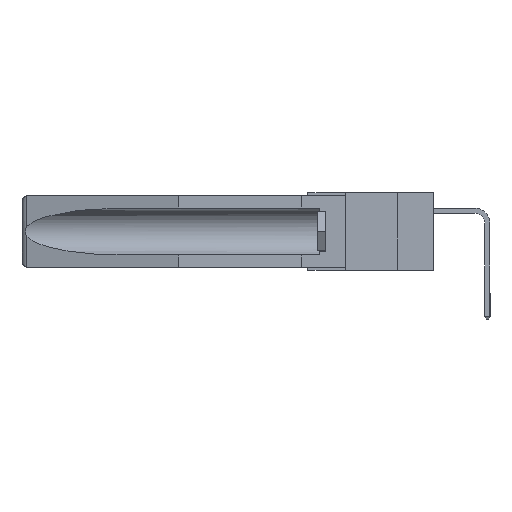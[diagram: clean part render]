
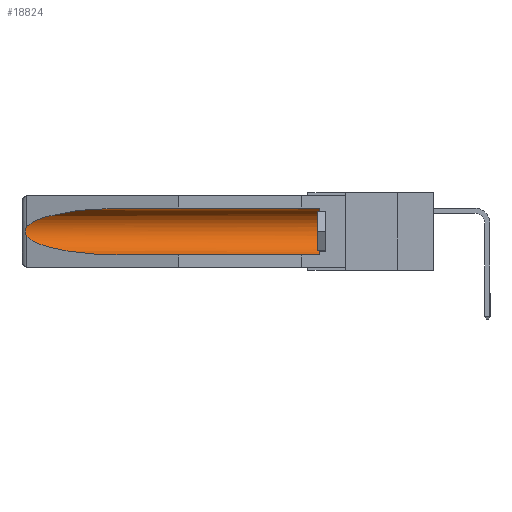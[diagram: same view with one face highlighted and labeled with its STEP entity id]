
A CAD part, left-side view. The second image highlights one B-rep face of the part: STEP entity #18824.
In plain terms, the highlighted cylindrical face has radius 2.857 mm (diameter 5.715 mm), a partial arc.
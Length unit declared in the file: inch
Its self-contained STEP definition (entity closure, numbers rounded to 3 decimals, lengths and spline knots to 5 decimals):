
#1118 = DIRECTION ( 'NONE',  ( 0., 1., 0. ) ) ;
#1363 = CARTESIAN_POINT ( 'NONE',  ( 0.26537, 1.52718, -0.19328 ) ) ;
#1457 = CARTESIAN_POINT ( 'NONE',  ( 0.25451, 1.48313, -0.24835 ) ) ;
#1878 = EDGE_CURVE ( 'NONE', #3964, #5398, #10526, .T. ) ;
#2089 = CARTESIAN_POINT ( 'NONE',  ( 0.26537, 1.52718, -0.19328 ) ) ;
#2339 = CARTESIAN_POINT ( 'NONE',  ( 0.26597, 1.5296, -0.19026 ) ) ;
#2630 = LINE ( 'NONE', #3405, #18219 ) ;
#3106 = VERTEX_POINT ( 'NONE', #24702 ) ;
#3405 = CARTESIAN_POINT ( 'NONE',  ( 0.155, -0.30754, -0.284 ) ) ;
#3619 = B_SPLINE_CURVE_WITH_KNOTS ( 'NONE', 3,
 ( #24090, #20144, #16199, #22167, #8186, #16105, #10196, #6261, #2339, #22258 ),
 .UNSPECIFIED., .F., .F.,
 ( 4, 2, 2, 2, 4 ),
 ( 0., 0.00029, 0.00058, 0.00087, 0.00117 ),
 .UNSPECIFIED. ) ;
#3673 = CARTESIAN_POINT ( 'NONE',  ( 0.155, 1.07973, -0.284 ) ) ;
#3964 = VERTEX_POINT ( 'NONE', #5039 ) ;
#5039 = CARTESIAN_POINT ( 'NONE',  ( 0.155, 1.07973, -0.059 ) ) ;
#5398 = VERTEX_POINT ( 'NONE', #8297 ) ;
#5708 = AXIS2_PLACEMENT_3D ( 'NONE', #14199, #18314, #12189 ) ;
#6104 = CYLINDRICAL_SURFACE ( 'NONE', #22093, 0.1125 ) ;
#6261 = CARTESIAN_POINT ( 'NONE',  ( 0.26655, 1.53094, -0.18657 ) ) ;
#6269 = CARTESIAN_POINT ( 'NONE',  ( 0.21114, 1.30732, -0.059 ) ) ;
#6389 = CARTESIAN_POINT ( 'NONE',  ( 0.155, -0.30754, -0.059 ) ) ;
#6666 =( BOUNDED_CURVE ( )  B_SPLINE_CURVE ( 3, ( #1363, #1457, #25586, #3673 ),
 .UNSPECIFIED., .F., .F. ) 
 B_SPLINE_CURVE_WITH_KNOTS ( ( 4, 4 ),
 ( 0.1948, 1.5708 ),
 .UNSPECIFIED. ) 
 CURVE ( )  GEOMETRIC_REPRESENTATION_ITEM ( )  RATIONAL_B_SPLINE_CURVE ( ( 1., 0.848, 0.848, 1. ) ) 
 REPRESENTATION_ITEM ( '' )  );
#7310 = DIRECTION ( 'NONE',  ( 0., 1., 0. ) ) ;
#8186 = CARTESIAN_POINT ( 'NONE',  ( 0.2675, 1.53308, -0.16763 ) ) ;
#8297 = CARTESIAN_POINT ( 'NONE',  ( 0.26537, 1.52718, -0.14972 ) ) ;
#8419 = DIRECTION ( 'NONE',  ( 0., 1., 0. ) ) ;
#8930 = FACE_OUTER_BOUND ( 'NONE', #15520, .T. ) ;
#9286 = ORIENTED_EDGE ( 'NONE', *, *, #22176, .T. ) ;
#10196 = CARTESIAN_POINT ( 'NONE',  ( 0.2673, 1.53269, -0.17917 ) ) ;
#10303 = CARTESIAN_POINT ( 'NONE',  ( 0.25451, 1.48313, -0.09465 ) ) ;
#10526 =( BOUNDED_CURVE ( )  B_SPLINE_CURVE ( 3, ( #21999, #6269, #10303, #11955 ),
 .UNSPECIFIED., .F., .F. ) 
 B_SPLINE_CURVE_WITH_KNOTS ( ( 4, 4 ),
 ( 4.71239, 6.08839 ),
 .UNSPECIFIED. ) 
 CURVE ( )  GEOMETRIC_REPRESENTATION_ITEM ( )  RATIONAL_B_SPLINE_CURVE ( ( 1., 0.848, 0.848, 1. ) ) 
 REPRESENTATION_ITEM ( '' )  );
#10573 = ORIENTED_EDGE ( 'NONE', *, *, #18373, .F. ) ;
#11500 = LINE ( 'NONE', #6389, #14938 ) ;
#11955 = CARTESIAN_POINT ( 'NONE',  ( 0.26537, 1.52718, -0.14972 ) ) ;
#12189 = DIRECTION ( 'NONE',  ( 0., 0., 1. ) ) ;
#12493 = EDGE_CURVE ( 'NONE', #25366, #17667, #6666, .T. ) ;
#12933 = EDGE_CURVE ( 'NONE', #3106, #3964, #11500, .T. ) ;
#14199 = CARTESIAN_POINT ( 'NONE',  ( 0.155, 0.126, -0.1715 ) ) ;
#14256 = ORIENTED_EDGE ( 'NONE', *, *, #12933, .T. ) ;
#14938 = VECTOR ( 'NONE', #8419, 39.37008 ) ;
#15520 = EDGE_LOOP ( 'NONE', ( #18788, #9286, #17429, #10573, #16141, #14256 ) ) ;
#16105 = CARTESIAN_POINT ( 'NONE',  ( 0.2675, 1.53308, -0.17534 ) ) ;
#16141 = ORIENTED_EDGE ( 'NONE', *, *, #20660, .T. ) ;
#16199 = CARTESIAN_POINT ( 'NONE',  ( 0.26654, 1.53092, -0.15636 ) ) ;
#17298 = CARTESIAN_POINT ( 'NONE',  ( 0.155, 0.126, -0.284 ) ) ;
#17429 = ORIENTED_EDGE ( 'NONE', *, *, #12493, .T. ) ;
#17509 = CIRCLE ( 'NONE', #5708, 0.1125 ) ;
#17667 = VERTEX_POINT ( 'NONE', #23056 ) ;
#17870 = VERTEX_POINT ( 'NONE', #17298 ) ;
#18219 = VECTOR ( 'NONE', #7310, 39.37008 ) ;
#18314 = DIRECTION ( 'NONE',  ( 0., -1., 0. ) ) ;
#18373 = EDGE_CURVE ( 'NONE', #17870, #17667, #2630, .T. ) ;
#18788 = ORIENTED_EDGE ( 'NONE', *, *, #1878, .T. ) ;
#18824 = ADVANCED_FACE ( 'NONE', ( #8930 ), #6104, .F. ) ;
#20144 = CARTESIAN_POINT ( 'NONE',  ( 0.26597, 1.52961, -0.15275 ) ) ;
#20660 = EDGE_CURVE ( 'NONE', #17870, #3106, #17509, .T. ) ;
#21772 = DIRECTION ( 'NONE',  ( 0., 0., 1. ) ) ;
#21999 = CARTESIAN_POINT ( 'NONE',  ( 0.155, 1.07973, -0.059 ) ) ;
#22093 = AXIS2_PLACEMENT_3D ( 'NONE', #23103, #1118, #21772 ) ;
#22167 = CARTESIAN_POINT ( 'NONE',  ( 0.2673, 1.5327, -0.16383 ) ) ;
#22176 = EDGE_CURVE ( 'NONE', #5398, #25366, #3619, .T. ) ;
#22258 = CARTESIAN_POINT ( 'NONE',  ( 0.26537, 1.52718, -0.19328 ) ) ;
#23056 = CARTESIAN_POINT ( 'NONE',  ( 0.155, 1.07973, -0.284 ) ) ;
#23103 = CARTESIAN_POINT ( 'NONE',  ( 0.155, -0.30754, -0.1715 ) ) ;
#24090 = CARTESIAN_POINT ( 'NONE',  ( 0.26537, 1.52718, -0.14972 ) ) ;
#24702 = CARTESIAN_POINT ( 'NONE',  ( 0.155, 0.126, -0.059 ) ) ;
#25366 = VERTEX_POINT ( 'NONE', #2089 ) ;
#25586 = CARTESIAN_POINT ( 'NONE',  ( 0.21114, 1.30732, -0.284 ) ) ;
